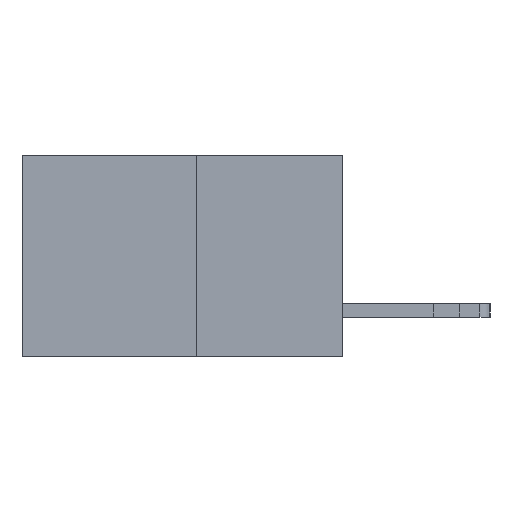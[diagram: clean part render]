
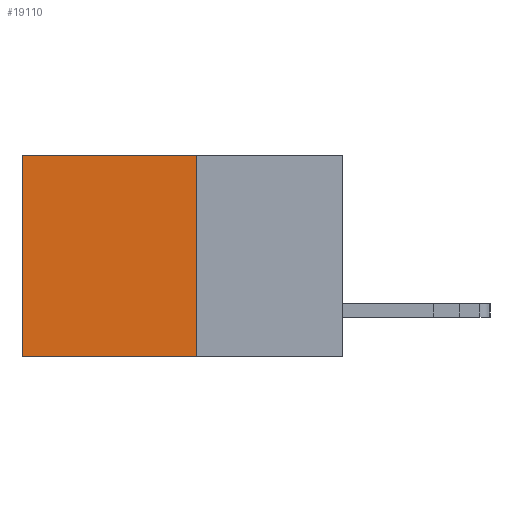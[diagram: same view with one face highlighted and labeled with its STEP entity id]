
A CAD part, left-side view. The second image highlights one B-rep face of the part: STEP entity #19110.
In plain terms, the highlighted planar face has unit normal (-1, 0, 0).
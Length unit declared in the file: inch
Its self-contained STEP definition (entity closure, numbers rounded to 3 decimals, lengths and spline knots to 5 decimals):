
#65 = CARTESIAN_POINT ( 'NONE',  ( 0.277, 0.27, 0. ) ) ;
#844 = FACE_OUTER_BOUND ( 'NONE', #7071, .T. ) ;
#969 = CARTESIAN_POINT ( 'NONE',  ( 0.277, 0.27, -0.37 ) ) ;
#1300 = LINE ( 'NONE', #19633, #18363 ) ;
#1483 = DIRECTION ( 'NONE',  ( 0., 0., -1. ) ) ;
#1887 = EDGE_CURVE ( 'NONE', #3780, #18874, #5018, .T. ) ;
#2120 = VERTEX_POINT ( 'NONE', #8413 ) ;
#2582 = PLANE ( 'NONE',  #19870 ) ;
#2604 = VERTEX_POINT ( 'NONE', #21152 ) ;
#3099 = DIRECTION ( 'NONE',  ( 0., 1., 0. ) ) ;
#3780 = VERTEX_POINT ( 'NONE', #969 ) ;
#4173 = LINE ( 'NONE', #65, #8104 ) ;
#4265 = LINE ( 'NONE', #15828, #21371 ) ;
#4369 = EDGE_CURVE ( 'NONE', #2120, #3780, #4265, .T. ) ;
#5018 = LINE ( 'NONE', #11856, #17235 ) ;
#5438 = ORIENTED_EDGE ( 'NONE', *, *, #1887, .F. ) ;
#5921 = CARTESIAN_POINT ( 'NONE',  ( 0.277, 0.27, -0.37 ) ) ;
#6965 = CARTESIAN_POINT ( 'NONE',  ( 0.277, 0.59, -0.37 ) ) ;
#7071 = EDGE_LOOP ( 'NONE', ( #15151, #5438, #9276, #20811 ) ) ;
#7612 = DIRECTION ( 'NONE',  ( 0., 0., -1. ) ) ;
#8104 = VECTOR ( 'NONE', #13413, 39.37008 ) ;
#8413 = CARTESIAN_POINT ( 'NONE',  ( 0.277, 0.27, 0. ) ) ;
#9276 = ORIENTED_EDGE ( 'NONE', *, *, #4369, .F. ) ;
#11856 = CARTESIAN_POINT ( 'NONE',  ( 0.277, 0.27, -0.37 ) ) ;
#13413 = DIRECTION ( 'NONE',  ( 0., 1., 0. ) ) ;
#14170 = DIRECTION ( 'NONE',  ( 0., 0., -1. ) ) ;
#15151 = ORIENTED_EDGE ( 'NONE', *, *, #19954, .T. ) ;
#15828 = CARTESIAN_POINT ( 'NONE',  ( 0.277, 0.27, -0.37 ) ) ;
#17235 = VECTOR ( 'NONE', #3099, 39.37008 ) ;
#17530 = DIRECTION ( 'NONE',  ( 1., 0., 0. ) ) ;
#18363 = VECTOR ( 'NONE', #1483, 39.37008 ) ;
#18755 = EDGE_CURVE ( 'NONE', #2120, #2604, #4173, .T. ) ;
#18874 = VERTEX_POINT ( 'NONE', #6965 ) ;
#19110 = ADVANCED_FACE ( 'NONE', ( #844 ), #2582, .F. ) ;
#19633 = CARTESIAN_POINT ( 'NONE',  ( 0.277, 0.59, -0.37 ) ) ;
#19870 = AXIS2_PLACEMENT_3D ( 'NONE', #5921, #17530, #7612 ) ;
#19954 = EDGE_CURVE ( 'NONE', #2604, #18874, #1300, .T. ) ;
#20811 = ORIENTED_EDGE ( 'NONE', *, *, #18755, .T. ) ;
#21152 = CARTESIAN_POINT ( 'NONE',  ( 0.277, 0.59, 0. ) ) ;
#21371 = VECTOR ( 'NONE', #14170, 39.37008 ) ;
